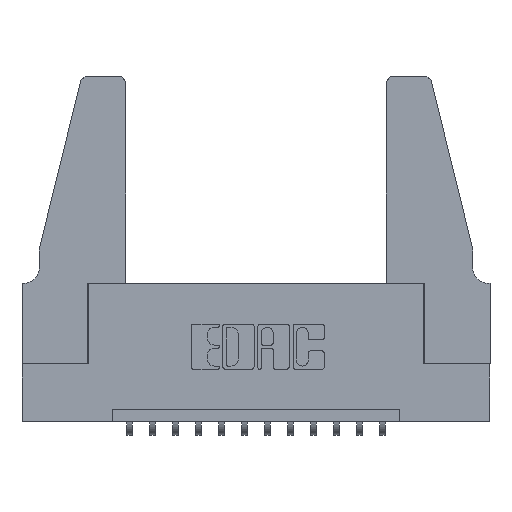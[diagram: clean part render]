
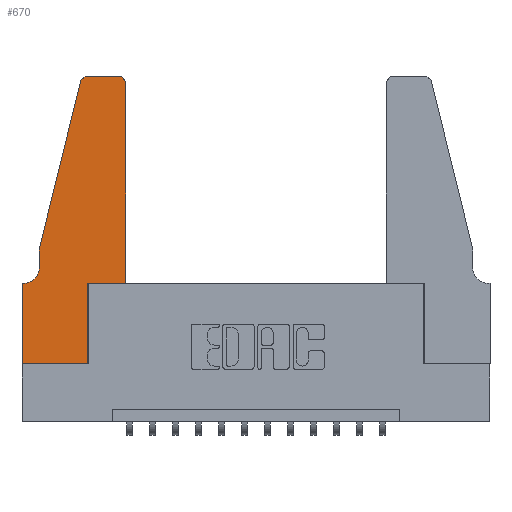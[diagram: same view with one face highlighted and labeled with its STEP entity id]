
A CAD part, top view. The second image highlights one B-rep face of the part: STEP entity #670.
In plain terms, the highlighted planar face has unit normal (0, 0, 1).
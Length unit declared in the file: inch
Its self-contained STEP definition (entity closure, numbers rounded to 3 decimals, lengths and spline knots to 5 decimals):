
#95 = PLANE ( 'NONE',  #1068 ) ;
#116 = FACE_OUTER_BOUND ( 'NONE', #2662, .T. ) ;
#147 = DIRECTION ( 'NONE',  ( 1., 0., 0. ) ) ;
#309 = EDGE_CURVE ( 'NONE', #1920, #4417, #13999, .T. ) ;
#331 = CARTESIAN_POINT ( 'NONE',  ( 0.4505, 0.35, 0.37 ) ) ;
#623 = CARTESIAN_POINT ( 'NONE',  ( 0., 0.35, 0.37 ) ) ;
#670 = ADVANCED_FACE ( 'NONE', ( #116 ), #95, .T. ) ;
#817 = LINE ( 'NONE', #12990, #13039 ) ;
#1068 = AXIS2_PLACEMENT_3D ( 'NONE', #9532, #8481, #5026 ) ;
#1285 = DIRECTION ( 'NONE',  ( -1., 0., 0. ) ) ;
#1485 = CARTESIAN_POINT ( 'NONE',  ( 0.2865, 0., 0.37 ) ) ;
#1595 = VECTOR ( 'NONE', #14455, 39.37008 ) ;
#1776 = VECTOR ( 'NONE', #2411, 39.37008 ) ;
#1854 = VECTOR ( 'NONE', #7777, 39.37008 ) ;
#1920 = VERTEX_POINT ( 'NONE', #14030 ) ;
#2332 = ORIENTED_EDGE ( 'NONE', *, *, #6016, .T. ) ;
#2411 = DIRECTION ( 'NONE',  ( 0., -1., 0. ) ) ;
#2543 = CIRCLE ( 'NONE', #6302, 0.03 ) ;
#2577 = CARTESIAN_POINT ( 'NONE',  ( 0.4205, 1.25, 0.37 ) ) ;
#2639 = CIRCLE ( 'NONE', #14133, 0.03 ) ;
#2662 = EDGE_LOOP ( 'NONE', ( #4433, #9665, #12185, #4294, #2332, #13634, #7864, #14944, #10149, #4851, #3096, #12875 ) ) ;
#2722 = DIRECTION ( 'NONE',  ( 0., 1., 0. ) ) ;
#3027 = CIRCLE ( 'NONE', #4605, 0.07 ) ;
#3030 = CARTESIAN_POINT ( 'NONE',  ( 0., 0., 0.37 ) ) ;
#3096 = ORIENTED_EDGE ( 'NONE', *, *, #13730, .T. ) ;
#3376 = CARTESIAN_POINT ( 'NONE',  ( 0.0055, 0.42, 0.37 ) ) ;
#3546 = LINE ( 'NONE', #5405, #1854 ) ;
#3592 = CARTESIAN_POINT ( 'NONE',  ( 0.25487, 1.22718, 0.37 ) ) ;
#3816 = CARTESIAN_POINT ( 'NONE',  ( 0.0755, 0.5, 0.37 ) ) ;
#3822 = LINE ( 'NONE', #3816, #1776 ) ;
#3876 = CARTESIAN_POINT ( 'NONE',  ( 0.4505, 0.35, 0.37 ) ) ;
#3941 = EDGE_CURVE ( 'NONE', #11586, #1920, #8254, .T. ) ;
#4294 = ORIENTED_EDGE ( 'NONE', *, *, #4359, .T. ) ;
#4359 = EDGE_CURVE ( 'NONE', #12158, #11940, #3822, .T. ) ;
#4417 = VERTEX_POINT ( 'NONE', #1485 ) ;
#4433 = ORIENTED_EDGE ( 'NONE', *, *, #11975, .T. ) ;
#4554 = DIRECTION ( 'NONE',  ( 0., 0., -1. ) ) ;
#4605 = AXIS2_PLACEMENT_3D ( 'NONE', #3376, #4554, #10352 ) ;
#4632 = VERTEX_POINT ( 'NONE', #10120 ) ;
#4747 = CARTESIAN_POINT ( 'NONE',  ( 0.4205, 1.22, 0.37 ) ) ;
#4767 = LINE ( 'NONE', #331, #12170 ) ;
#4851 = ORIENTED_EDGE ( 'NONE', *, *, #9346, .T. ) ;
#5026 = DIRECTION ( 'NONE',  ( 1., 0., 0. ) ) ;
#5051 = LINE ( 'NONE', #9962, #5977 ) ;
#5405 = CARTESIAN_POINT ( 'NONE',  ( 0.2605, 1.25, 0.37 ) ) ;
#5497 = CARTESIAN_POINT ( 'NONE',  ( 0.0755, 0.5, 0.37 ) ) ;
#5639 = VERTEX_POINT ( 'NONE', #2577 ) ;
#5703 = CARTESIAN_POINT ( 'NONE',  ( 0.0755, 0.42, 0.37 ) ) ;
#5977 = VECTOR ( 'NONE', #9855, 39.37008 ) ;
#6016 = EDGE_CURVE ( 'NONE', #11940, #6336, #3027, .T. ) ;
#6152 = DIRECTION ( 'NONE',  ( -0.239, -0.971, 0. ) ) ;
#6262 = EDGE_CURVE ( 'NONE', #4417, #8680, #5051, .T. ) ;
#6302 = AXIS2_PLACEMENT_3D ( 'NONE', #7331, #9725, #147 ) ;
#6336 = VERTEX_POINT ( 'NONE', #7630 ) ;
#6545 = DIRECTION ( 'NONE',  ( 1., 0., 0. ) ) ;
#7158 = DIRECTION ( 'NONE',  ( 1., 0., 0. ) ) ;
#7171 = VECTOR ( 'NONE', #6545, 39.37008 ) ;
#7331 = CARTESIAN_POINT ( 'NONE',  ( 0.284, 1.22, 0.37 ) ) ;
#7630 = CARTESIAN_POINT ( 'NONE',  ( 0.0055, 0.35, 0.37 ) ) ;
#7777 = DIRECTION ( 'NONE',  ( -1., 0., 0. ) ) ;
#7864 = ORIENTED_EDGE ( 'NONE', *, *, #3941, .T. ) ;
#8177 = VERTEX_POINT ( 'NONE', #3592 ) ;
#8219 = LINE ( 'NONE', #3876, #12110 ) ;
#8254 = LINE ( 'NONE', #13372, #1595 ) ;
#8481 = DIRECTION ( 'NONE',  ( 0., 0., 1. ) ) ;
#8680 = VERTEX_POINT ( 'NONE', #9859 ) ;
#8782 = DIRECTION ( 'NONE',  ( 1., 0., 0. ) ) ;
#8993 = EDGE_CURVE ( 'NONE', #11339, #8177, #2543, .T. ) ;
#9036 = EDGE_CURVE ( 'NONE', #6336, #11586, #14754, .T. ) ;
#9346 = EDGE_CURVE ( 'NONE', #8680, #4632, #8219, .T. ) ;
#9532 = CARTESIAN_POINT ( 'NONE',  ( 0., 0.35, 0.37 ) ) ;
#9665 = ORIENTED_EDGE ( 'NONE', *, *, #8993, .T. ) ;
#9725 = DIRECTION ( 'NONE',  ( 0., 0., 1. ) ) ;
#9850 = EDGE_CURVE ( 'NONE', #14861, #5639, #2639, .T. ) ;
#9855 = DIRECTION ( 'NONE',  ( 0., 1., 0. ) ) ;
#9859 = CARTESIAN_POINT ( 'NONE',  ( 0.2865, 0.35, 0.37 ) ) ;
#9961 = VECTOR ( 'NONE', #1285, 39.37008 ) ;
#9962 = CARTESIAN_POINT ( 'NONE',  ( 0.2865, 0.35, 0.37 ) ) ;
#10120 = CARTESIAN_POINT ( 'NONE',  ( 0.4505, 0.35, 0.37 ) ) ;
#10149 = ORIENTED_EDGE ( 'NONE', *, *, #6262, .T. ) ;
#10352 = DIRECTION ( 'NONE',  ( -1., 0., 0. ) ) ;
#11339 = VERTEX_POINT ( 'NONE', #13707 ) ;
#11586 = VERTEX_POINT ( 'NONE', #623 ) ;
#11940 = VERTEX_POINT ( 'NONE', #5703 ) ;
#11975 = EDGE_CURVE ( 'NONE', #5639, #11339, #3546, .T. ) ;
#12110 = VECTOR ( 'NONE', #8782, 39.37008 ) ;
#12158 = VERTEX_POINT ( 'NONE', #5497 ) ;
#12170 = VECTOR ( 'NONE', #2722, 39.37008 ) ;
#12185 = ORIENTED_EDGE ( 'NONE', *, *, #15142, .T. ) ;
#12875 = ORIENTED_EDGE ( 'NONE', *, *, #9850, .T. ) ;
#12990 = CARTESIAN_POINT ( 'NONE',  ( 0.0755, 0.5, 0.37 ) ) ;
#13039 = VECTOR ( 'NONE', #6152, 39.37008 ) ;
#13086 = CARTESIAN_POINT ( 'NONE',  ( 0.0755, 0.35, 0.37 ) ) ;
#13372 = CARTESIAN_POINT ( 'NONE',  ( 0., 0., 0.37 ) ) ;
#13634 = ORIENTED_EDGE ( 'NONE', *, *, #9036, .T. ) ;
#13707 = CARTESIAN_POINT ( 'NONE',  ( 0.284, 1.25, 0.37 ) ) ;
#13730 = EDGE_CURVE ( 'NONE', #4632, #14861, #4767, .T. ) ;
#13999 = LINE ( 'NONE', #3030, #7171 ) ;
#14000 = CARTESIAN_POINT ( 'NONE',  ( 0.4505, 1.22, 0.37 ) ) ;
#14030 = CARTESIAN_POINT ( 'NONE',  ( 0., 0., 0.37 ) ) ;
#14133 = AXIS2_PLACEMENT_3D ( 'NONE', #4747, #14228, #7158 ) ;
#14228 = DIRECTION ( 'NONE',  ( 0., 0., 1. ) ) ;
#14455 = DIRECTION ( 'NONE',  ( 0., -1., 0. ) ) ;
#14754 = LINE ( 'NONE', #13086, #9961 ) ;
#14861 = VERTEX_POINT ( 'NONE', #14000 ) ;
#14944 = ORIENTED_EDGE ( 'NONE', *, *, #309, .T. ) ;
#15142 = EDGE_CURVE ( 'NONE', #8177, #12158, #817, .T. ) ;
